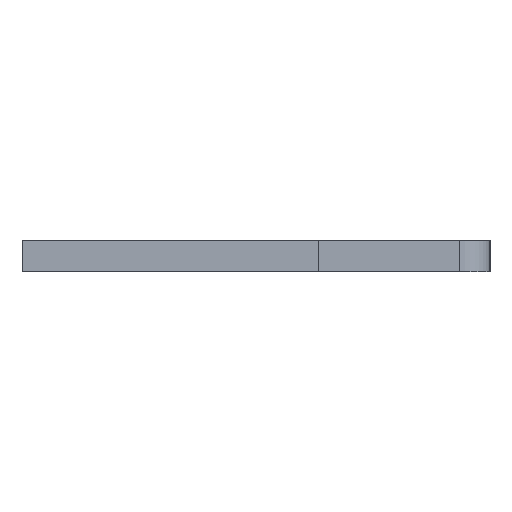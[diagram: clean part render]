
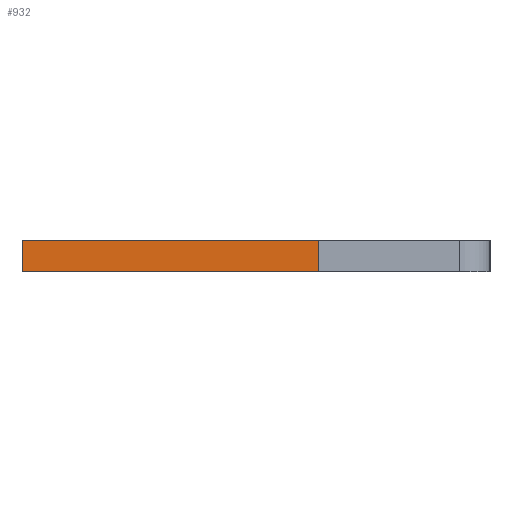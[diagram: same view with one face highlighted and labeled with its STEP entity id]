
A CAD part, left-side view. The second image highlights one B-rep face of the part: STEP entity #932.
In plain terms, the highlighted face is planar.
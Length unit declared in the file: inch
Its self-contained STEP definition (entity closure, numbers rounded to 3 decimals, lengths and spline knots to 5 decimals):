
#148 = FACE_OUTER_BOUND ( 'NONE', #292, .T. ) ;
#292 = EDGE_LOOP ( 'NONE', ( #1964, #673, #1723, #469 ) ) ;
#441 = CARTESIAN_POINT ( 'NONE',  ( 0.01, 0.15, -0.04 ) ) ;
#467 = EDGE_CURVE ( 'NONE', #2408, #1234, #1247, .T. ) ;
#469 = ORIENTED_EDGE ( 'NONE', *, *, #2576, .T. ) ;
#582 = CARTESIAN_POINT ( 'NONE',  ( 0.01, -0.04, -0.04 ) ) ;
#659 = DIRECTION ( 'NONE',  ( -1., 0., 0. ) ) ;
#673 = ORIENTED_EDGE ( 'NONE', *, *, #1052, .F. ) ;
#853 = CARTESIAN_POINT ( 'NONE',  ( -0.01, 0.15, -0.04 ) ) ;
#876 = DIRECTION ( 'NONE',  ( 0., 1., 0. ) ) ;
#913 = VERTEX_POINT ( 'NONE', #853 ) ;
#932 = ADVANCED_FACE ( 'NONE', ( #148 ), #1895, .F. ) ;
#1052 = EDGE_CURVE ( 'NONE', #1234, #913, #1402, .T. ) ;
#1121 = EDGE_CURVE ( 'NONE', #1554, #913, #1533, .T. ) ;
#1234 = VERTEX_POINT ( 'NONE', #1288 ) ;
#1247 = LINE ( 'NONE', #2480, #2088 ) ;
#1255 = VECTOR ( 'NONE', #659, 39.37008 ) ;
#1288 = CARTESIAN_POINT ( 'NONE',  ( 0.01, 0.15, -0.04 ) ) ;
#1402 = LINE ( 'NONE', #441, #1255 ) ;
#1403 = DIRECTION ( 'NONE',  ( -1., 0., 0. ) ) ;
#1468 = AXIS2_PLACEMENT_3D ( 'NONE', #1687, #2286, #2511 ) ;
#1533 = LINE ( 'NONE', #1879, #2020 ) ;
#1554 = VERTEX_POINT ( 'NONE', #1915 ) ;
#1687 = CARTESIAN_POINT ( 'NONE',  ( 0.01, 0.15, -0.04 ) ) ;
#1723 = ORIENTED_EDGE ( 'NONE', *, *, #467, .F. ) ;
#1835 = DIRECTION ( 'NONE',  ( 0., 1., 0. ) ) ;
#1879 = CARTESIAN_POINT ( 'NONE',  ( -0.01, 0.15, -0.04 ) ) ;
#1895 = PLANE ( 'NONE',  #1468 ) ;
#1915 = CARTESIAN_POINT ( 'NONE',  ( -0.01, -0.04, -0.04 ) ) ;
#1964 = ORIENTED_EDGE ( 'NONE', *, *, #1121, .T. ) ;
#1989 = VECTOR ( 'NONE', #1403, 39.37008 ) ;
#2020 = VECTOR ( 'NONE', #876, 39.37008 ) ;
#2088 = VECTOR ( 'NONE', #1835, 39.37008 ) ;
#2286 = DIRECTION ( 'NONE',  ( 0., 0., 1. ) ) ;
#2400 = LINE ( 'NONE', #582, #1989 ) ;
#2408 = VERTEX_POINT ( 'NONE', #2573 ) ;
#2480 = CARTESIAN_POINT ( 'NONE',  ( 0.01, 0.15, -0.04 ) ) ;
#2511 = DIRECTION ( 'NONE',  ( 1., 0., 0. ) ) ;
#2573 = CARTESIAN_POINT ( 'NONE',  ( 0.01, -0.04, -0.04 ) ) ;
#2576 = EDGE_CURVE ( 'NONE', #2408, #1554, #2400, .T. ) ;
